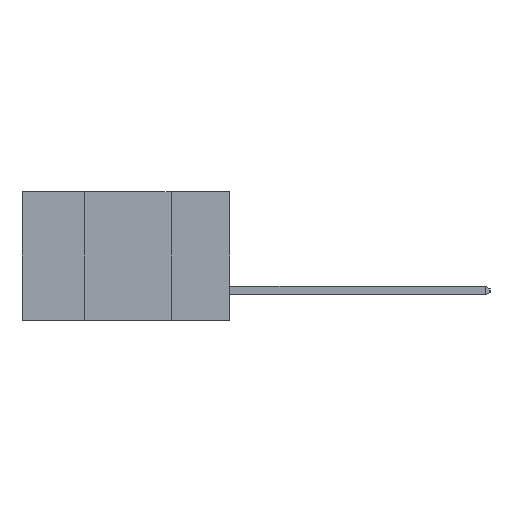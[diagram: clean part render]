
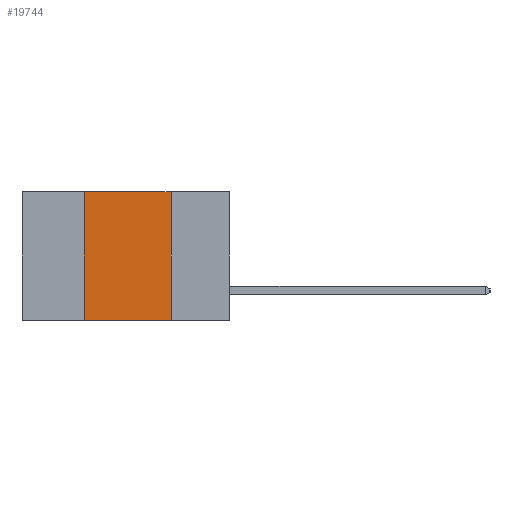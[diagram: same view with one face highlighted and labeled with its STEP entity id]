
A CAD part, left-side view. The second image highlights one B-rep face of the part: STEP entity #19744.
In plain terms, the highlighted planar face has unit normal (-1, 0, 0).
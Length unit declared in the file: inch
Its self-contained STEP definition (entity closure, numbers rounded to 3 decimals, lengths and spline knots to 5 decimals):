
#304 = VERTEX_POINT ( 'NONE', #2850 ) ;
#2012 = PLANE ( 'NONE',  #17687 ) ;
#2850 = CARTESIAN_POINT ( 'NONE',  ( 0., 0.17, -0.37 ) ) ;
#4273 = CARTESIAN_POINT ( 'NONE',  ( 0., 0.6, -0.37 ) ) ;
#4504 = EDGE_CURVE ( 'NONE', #13214, #304, #10608, .T. ) ;
#4826 = VECTOR ( 'NONE', #25513, 39.37008 ) ;
#5267 = DIRECTION ( 'NONE',  ( 0., 0., 1. ) ) ;
#6285 = DIRECTION ( 'NONE',  ( 1., 0., 0. ) ) ;
#6973 = CARTESIAN_POINT ( 'NONE',  ( 0., 0.17, 0. ) ) ;
#7431 = LINE ( 'NONE', #26407, #22419 ) ;
#7538 = EDGE_CURVE ( 'NONE', #19608, #304, #17422, .T. ) ;
#7679 = EDGE_CURVE ( 'NONE', #22847, #13214, #12738, .T. ) ;
#8496 = ORIENTED_EDGE ( 'NONE', *, *, #24776, .F. ) ;
#8889 = CARTESIAN_POINT ( 'NONE',  ( 0., 0.42, 0. ) ) ;
#9561 = CARTESIAN_POINT ( 'NONE',  ( 0., 0.17, 0. ) ) ;
#10608 = LINE ( 'NONE', #6973, #11274 ) ;
#11274 = VECTOR ( 'NONE', #26091, 39.37008 ) ;
#12051 = VECTOR ( 'NONE', #21667, 39.37008 ) ;
#12437 = FACE_OUTER_BOUND ( 'NONE', #19190, .T. ) ;
#12738 = LINE ( 'NONE', #13129, #12051 ) ;
#13129 = CARTESIAN_POINT ( 'NONE',  ( 0., 0.6, 0. ) ) ;
#13214 = VERTEX_POINT ( 'NONE', #9561 ) ;
#13774 = ORIENTED_EDGE ( 'NONE', *, *, #7679, .F. ) ;
#14350 = ORIENTED_EDGE ( 'NONE', *, *, #7538, .T. ) ;
#16566 = CARTESIAN_POINT ( 'NONE',  ( 0., 0.42, -0.37 ) ) ;
#17422 = LINE ( 'NONE', #4273, #4826 ) ;
#17687 = AXIS2_PLACEMENT_3D ( 'NONE', #23215, #6285, #21150 ) ;
#19190 = EDGE_LOOP ( 'NONE', ( #20072, #13774, #8496, #14350 ) ) ;
#19608 = VERTEX_POINT ( 'NONE', #16566 ) ;
#19744 = ADVANCED_FACE ( 'NONE', ( #12437 ), #2012, .F. ) ;
#20072 = ORIENTED_EDGE ( 'NONE', *, *, #4504, .F. ) ;
#21150 = DIRECTION ( 'NONE',  ( 0., 0., -1. ) ) ;
#21667 = DIRECTION ( 'NONE',  ( 0., -1., 0. ) ) ;
#22419 = VECTOR ( 'NONE', #5267, 39.37008 ) ;
#22847 = VERTEX_POINT ( 'NONE', #8889 ) ;
#23215 = CARTESIAN_POINT ( 'NONE',  ( 0., 0.6, 0. ) ) ;
#24776 = EDGE_CURVE ( 'NONE', #19608, #22847, #7431, .T. ) ;
#25513 = DIRECTION ( 'NONE',  ( 0., -1., 0. ) ) ;
#26091 = DIRECTION ( 'NONE',  ( 0., 0., -1. ) ) ;
#26407 = CARTESIAN_POINT ( 'NONE',  ( 0., 0.42, 0. ) ) ;
